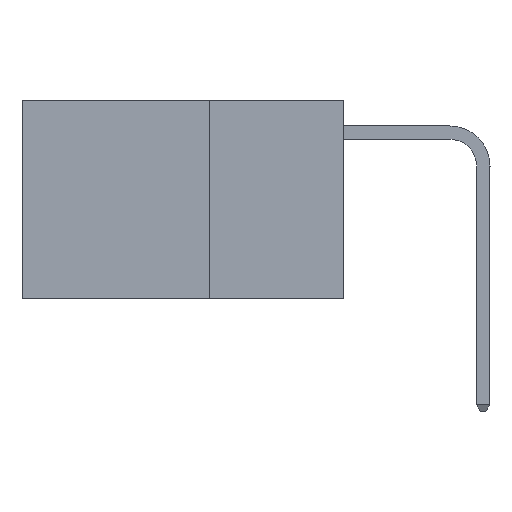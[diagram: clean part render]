
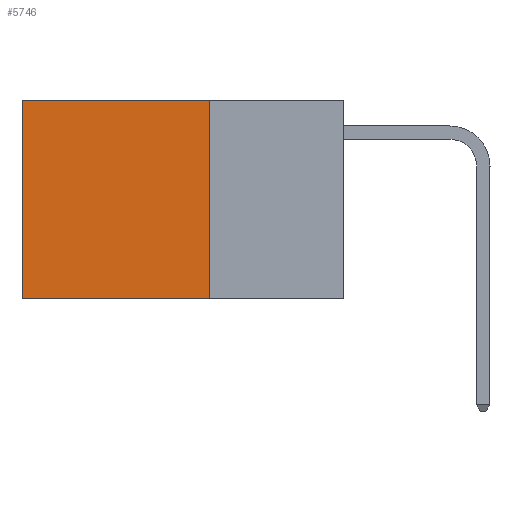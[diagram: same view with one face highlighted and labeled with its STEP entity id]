
A CAD part, left-side view. The second image highlights one B-rep face of the part: STEP entity #5746.
In plain terms, the highlighted planar face has unit normal (-1, 0, 0).
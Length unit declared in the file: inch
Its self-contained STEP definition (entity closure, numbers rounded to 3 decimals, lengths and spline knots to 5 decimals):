
#487 = CARTESIAN_POINT ( 'NONE',  ( 0.2625, 0.6, 0. ) ) ;
#853 = EDGE_CURVE ( 'NONE', #15212, #5338, #11858, .T. ) ;
#1138 = ORIENTED_EDGE ( 'NONE', *, *, #13543, .T. ) ;
#2185 = EDGE_LOOP ( 'NONE', ( #7396, #3492, #14324, #1138 ) ) ;
#2359 = DIRECTION ( 'NONE',  ( 0., 1., 0. ) ) ;
#3492 = ORIENTED_EDGE ( 'NONE', *, *, #853, .F. ) ;
#3601 = VERTEX_POINT ( 'NONE', #11310 ) ;
#3805 = VECTOR ( 'NONE', #7207, 39.37008 ) ;
#5338 = VERTEX_POINT ( 'NONE', #26007 ) ;
#5746 = ADVANCED_FACE ( 'NONE', ( #26931 ), #16690, .F. ) ;
#6378 = DIRECTION ( 'NONE',  ( 0., 0., -1. ) ) ;
#6715 = CARTESIAN_POINT ( 'NONE',  ( 0.2625, 0.25, 0. ) ) ;
#6911 = CARTESIAN_POINT ( 'NONE',  ( 0.2625, 0.25, -0.37 ) ) ;
#7207 = DIRECTION ( 'NONE',  ( 0., 0., -1. ) ) ;
#7336 = LINE ( 'NONE', #8525, #24238 ) ;
#7396 = ORIENTED_EDGE ( 'NONE', *, *, #28193, .T. ) ;
#7981 = DIRECTION ( 'NONE',  ( 1., 0., 0. ) ) ;
#8525 = CARTESIAN_POINT ( 'NONE',  ( 0.2625, 0.25, 0. ) ) ;
#10352 = LINE ( 'NONE', #487, #3805 ) ;
#11310 = CARTESIAN_POINT ( 'NONE',  ( 0.2625, 0.6, 0. ) ) ;
#11858 = LINE ( 'NONE', #6911, #22940 ) ;
#13543 = EDGE_CURVE ( 'NONE', #22601, #3601, #14885, .T. ) ;
#13901 = DIRECTION ( 'NONE',  ( 0., 1., 0. ) ) ;
#14204 = VECTOR ( 'NONE', #13901, 39.37008 ) ;
#14324 = ORIENTED_EDGE ( 'NONE', *, *, #26164, .F. ) ;
#14885 = LINE ( 'NONE', #27113, #14204 ) ;
#15212 = VERTEX_POINT ( 'NONE', #25653 ) ;
#16690 = PLANE ( 'NONE',  #25521 ) ;
#22601 = VERTEX_POINT ( 'NONE', #6715 ) ;
#22940 = VECTOR ( 'NONE', #2359, 39.37008 ) ;
#23404 = DIRECTION ( 'NONE',  ( 0., 0., -1. ) ) ;
#24238 = VECTOR ( 'NONE', #6378, 39.37008 ) ;
#25521 = AXIS2_PLACEMENT_3D ( 'NONE', #27701, #7981, #23404 ) ;
#25653 = CARTESIAN_POINT ( 'NONE',  ( 0.2625, 0.25, -0.37 ) ) ;
#26007 = CARTESIAN_POINT ( 'NONE',  ( 0.2625, 0.6, -0.37 ) ) ;
#26164 = EDGE_CURVE ( 'NONE', #22601, #15212, #7336, .T. ) ;
#26931 = FACE_OUTER_BOUND ( 'NONE', #2185, .T. ) ;
#27113 = CARTESIAN_POINT ( 'NONE',  ( 0.2625, 0.25, 0. ) ) ;
#27701 = CARTESIAN_POINT ( 'NONE',  ( 0.2625, 0.25, 0. ) ) ;
#28193 = EDGE_CURVE ( 'NONE', #3601, #5338, #10352, .T. ) ;
